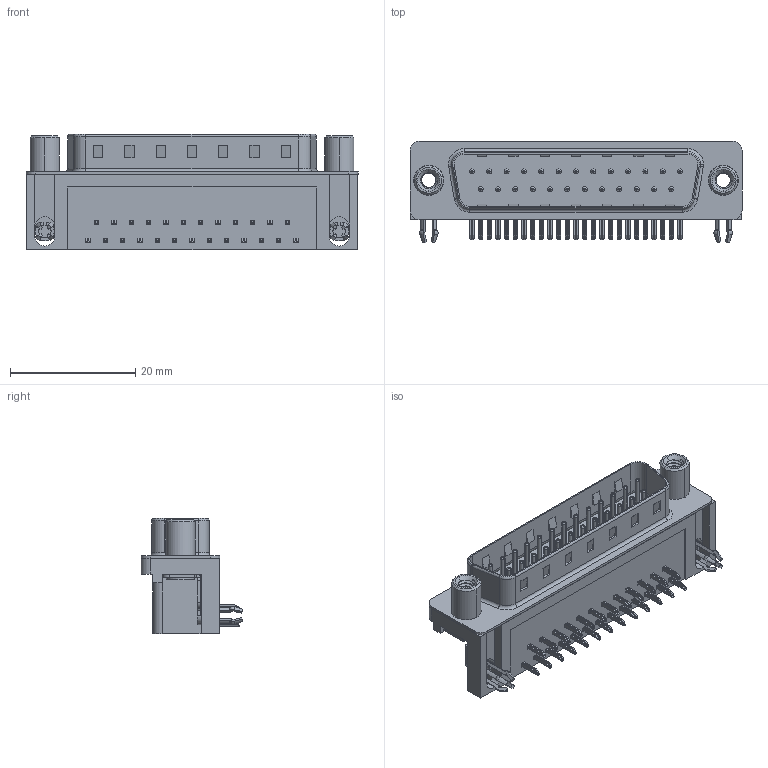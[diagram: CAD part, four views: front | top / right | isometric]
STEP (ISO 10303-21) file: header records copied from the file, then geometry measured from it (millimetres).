
FILE_DESCRIPTION (( 'STEP AP203' ), '1' );
FILE_NAME ('621-025-660-540.STEP', '2019-11-19T06:09:11', ( '' ), ( '' ), 'SwSTEP 2.0', 'SolidWorks 2016', '' );
FILE_SCHEMA (( 'CONFIG_CONTROL_DESIGN' ));
Length unit declared in the file: millimetre
Products named in the file (7): 621 Contact Top; 621 4 Prong Board Lock; 621-025-660-540; 621 Housing_25 Socket; 621 Shell_25 Socket; 621 Round Threaded Standoff; 621 Contact Bottom
Assembly tree (31 placements, depth 2):
  621-025-660-540
    621 Housing_25 Socket
    621 Shell_25 Socket
    621 Contact Bottom  x12
    621 Contact Top  x13
    621 4 Prong Board Lock  x2
    621 Round Threaded Standoff  x2
Bounding box: 53.04 x 16.25 x 18.4 mm (x, y, z)
Volume: 6447.6 mm3; surface area: 7956.6 mm2
Topology: 31 solids, 31 shells, 2377 faces, 5965 edges, 3705 vertices
Faces by surface type: plane 1439, cylinder 673, torus 197, cone 52, bspline 16
Entity records: 24770 total; most frequent: CARTESIAN_POINT 5693, DIRECTION 3731, ORIENTED_EDGE 3618, EDGE_CURVE 1809, AXIS2_PLACEMENT_3D 1249, LINE 1233, VECTOR 1233, VERTEX_POINT 1167
